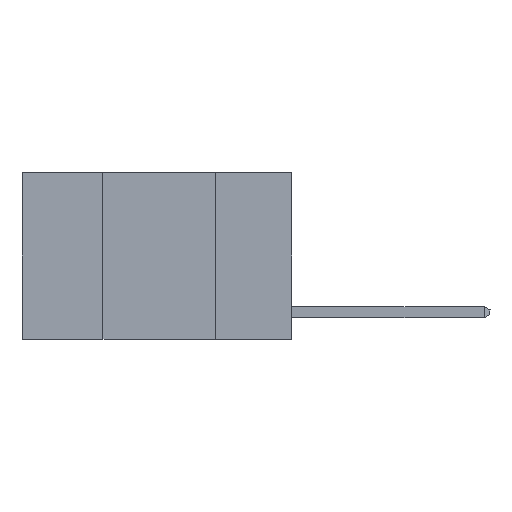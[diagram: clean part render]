
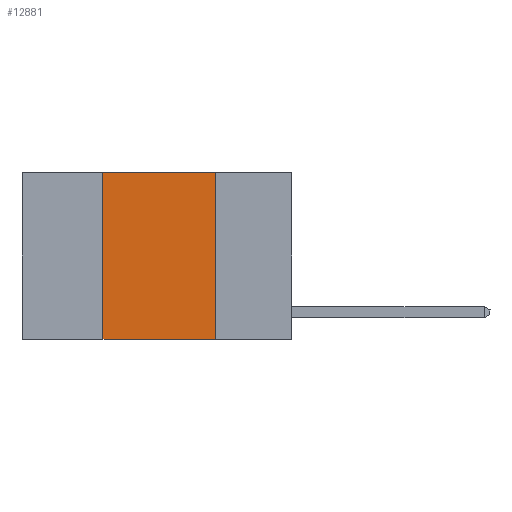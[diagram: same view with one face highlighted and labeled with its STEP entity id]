
A CAD part, left-side view. The second image highlights one B-rep face of the part: STEP entity #12881.
In plain terms, the highlighted planar face has unit normal (-1, 0, 0).
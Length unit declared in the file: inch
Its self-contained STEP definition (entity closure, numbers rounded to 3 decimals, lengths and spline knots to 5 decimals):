
#150 = EDGE_CURVE ( 'NONE', #13810, #17571, #326, .T. ) ;
#256 = EDGE_CURVE ( 'NONE', #24250, #17571, #9928, .T. ) ;
#326 = LINE ( 'NONE', #10524, #17398 ) ;
#991 = CARTESIAN_POINT ( 'NONE',  ( 0., 0.17, 0. ) ) ;
#1204 = VECTOR ( 'NONE', #7133, 39.37008 ) ;
#1854 = VERTEX_POINT ( 'NONE', #25586 ) ;
#2059 = DIRECTION ( 'NONE',  ( 0., -1., 0. ) ) ;
#2874 = ORIENTED_EDGE ( 'NONE', *, *, #7788, .F. ) ;
#5043 = CARTESIAN_POINT ( 'NONE',  ( 0., 0.6, 0. ) ) ;
#6184 = LINE ( 'NONE', #5043, #1204 ) ;
#6471 = ORIENTED_EDGE ( 'NONE', *, *, #150, .T. ) ;
#7133 = DIRECTION ( 'NONE',  ( 0., -1., 0. ) ) ;
#7788 = EDGE_CURVE ( 'NONE', #13810, #1854, #22740, .T. ) ;
#9710 = ORIENTED_EDGE ( 'NONE', *, *, #256, .F. ) ;
#9928 = LINE ( 'NONE', #21285, #25926 ) ;
#10219 = PLANE ( 'NONE',  #22827 ) ;
#10413 = CARTESIAN_POINT ( 'NONE',  ( 0., 0.42, -0.37 ) ) ;
#10524 = CARTESIAN_POINT ( 'NONE',  ( 0., 0.6, -0.37 ) ) ;
#12881 = ADVANCED_FACE ( 'NONE', ( #23129 ), #10219, .F. ) ;
#13810 = VERTEX_POINT ( 'NONE', #10413 ) ;
#15876 = EDGE_CURVE ( 'NONE', #1854, #24250, #6184, .T. ) ;
#16005 = ORIENTED_EDGE ( 'NONE', *, *, #15876, .F. ) ;
#16857 = VECTOR ( 'NONE', #26549, 39.37008 ) ;
#17398 = VECTOR ( 'NONE', #2059, 39.37008 ) ;
#17571 = VERTEX_POINT ( 'NONE', #22445 ) ;
#18484 = DIRECTION ( 'NONE',  ( 1., 0., 0. ) ) ;
#18872 = EDGE_LOOP ( 'NONE', ( #9710, #16005, #2874, #6471 ) ) ;
#20676 = CARTESIAN_POINT ( 'NONE',  ( 0., 0.6, 0. ) ) ;
#21285 = CARTESIAN_POINT ( 'NONE',  ( 0., 0.17, 0. ) ) ;
#22445 = CARTESIAN_POINT ( 'NONE',  ( 0., 0.17, -0.37 ) ) ;
#22740 = LINE ( 'NONE', #24148, #16857 ) ;
#22827 = AXIS2_PLACEMENT_3D ( 'NONE', #20676, #18484, #26556 ) ;
#23129 = FACE_OUTER_BOUND ( 'NONE', #18872, .T. ) ;
#23488 = DIRECTION ( 'NONE',  ( 0., 0., -1. ) ) ;
#24148 = CARTESIAN_POINT ( 'NONE',  ( 0., 0.42, 0. ) ) ;
#24250 = VERTEX_POINT ( 'NONE', #991 ) ;
#25586 = CARTESIAN_POINT ( 'NONE',  ( 0., 0.42, 0. ) ) ;
#25926 = VECTOR ( 'NONE', #23488, 39.37008 ) ;
#26549 = DIRECTION ( 'NONE',  ( 0., 0., 1. ) ) ;
#26556 = DIRECTION ( 'NONE',  ( 0., 0., -1. ) ) ;
